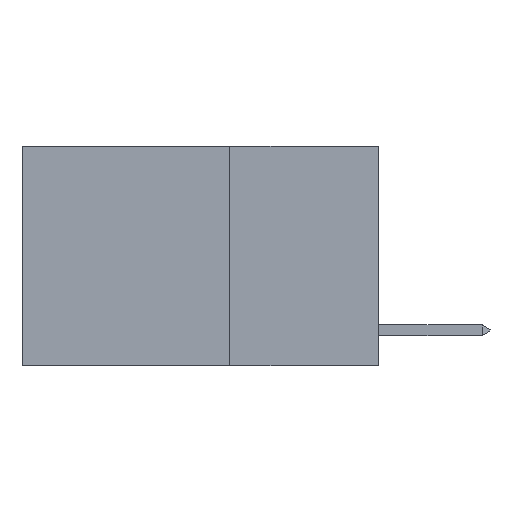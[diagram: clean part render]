
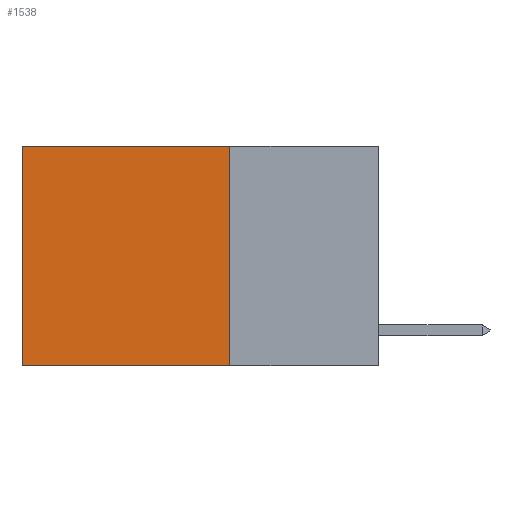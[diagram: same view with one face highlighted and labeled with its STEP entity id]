
A CAD part, left-side view. The second image highlights one B-rep face of the part: STEP entity #1538.
In plain terms, the highlighted planar face has unit normal (-1, 0, 0).
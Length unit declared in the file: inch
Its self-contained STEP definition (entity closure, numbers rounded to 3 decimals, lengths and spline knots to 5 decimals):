
#227 = CARTESIAN_POINT ( 'NONE',  ( 0.2625, 0.25, -0.37 ) ) ;
#251 = LINE ( 'NONE', #4106, #9109 ) ;
#510 = EDGE_CURVE ( 'NONE', #10621, #9238, #251, .T. ) ;
#785 = ORIENTED_EDGE ( 'NONE', *, *, #6155, .F. ) ;
#881 = DIRECTION ( 'NONE',  ( 0., 1., 0. ) ) ;
#1081 = LINE ( 'NONE', #10365, #2704 ) ;
#1084 = VERTEX_POINT ( 'NONE', #8723 ) ;
#1538 = ADVANCED_FACE ( 'NONE', ( #9565 ), #6943, .F. ) ;
#2236 = VECTOR ( 'NONE', #9667, 39.37008 ) ;
#2458 = LINE ( 'NONE', #8044, #3134 ) ;
#2628 = AXIS2_PLACEMENT_3D ( 'NONE', #7135, #2821, #6001 ) ;
#2704 = VECTOR ( 'NONE', #881, 39.37008 ) ;
#2821 = DIRECTION ( 'NONE',  ( 1., 0., 0. ) ) ;
#3134 = VECTOR ( 'NONE', #11124, 39.37008 ) ;
#3176 = EDGE_CURVE ( 'NONE', #6119, #1084, #2458, .T. ) ;
#4106 = CARTESIAN_POINT ( 'NONE',  ( 0.2625, 0.6, 0. ) ) ;
#5242 = ORIENTED_EDGE ( 'NONE', *, *, #6994, .T. ) ;
#6001 = DIRECTION ( 'NONE',  ( 0., 0., -1. ) ) ;
#6119 = VERTEX_POINT ( 'NONE', #10508 ) ;
#6155 = EDGE_CURVE ( 'NONE', #1084, #9238, #13558, .T. ) ;
#6943 = PLANE ( 'NONE',  #2628 ) ;
#6994 = EDGE_CURVE ( 'NONE', #6119, #10621, #1081, .T. ) ;
#7135 = CARTESIAN_POINT ( 'NONE',  ( 0.2625, 0.25, 0. ) ) ;
#7922 = ORIENTED_EDGE ( 'NONE', *, *, #510, .T. ) ;
#8044 = CARTESIAN_POINT ( 'NONE',  ( 0.2625, 0.25, 0. ) ) ;
#8723 = CARTESIAN_POINT ( 'NONE',  ( 0.2625, 0.25, -0.37 ) ) ;
#8806 = EDGE_LOOP ( 'NONE', ( #7922, #785, #10572, #5242 ) ) ;
#9109 = VECTOR ( 'NONE', #12484, 39.37008 ) ;
#9238 = VERTEX_POINT ( 'NONE', #9365 ) ;
#9365 = CARTESIAN_POINT ( 'NONE',  ( 0.2625, 0.6, -0.37 ) ) ;
#9565 = FACE_OUTER_BOUND ( 'NONE', #8806, .T. ) ;
#9667 = DIRECTION ( 'NONE',  ( 0., 1., 0. ) ) ;
#10365 = CARTESIAN_POINT ( 'NONE',  ( 0.2625, 0.25, 0. ) ) ;
#10508 = CARTESIAN_POINT ( 'NONE',  ( 0.2625, 0.25, 0. ) ) ;
#10572 = ORIENTED_EDGE ( 'NONE', *, *, #3176, .F. ) ;
#10621 = VERTEX_POINT ( 'NONE', #12940 ) ;
#11124 = DIRECTION ( 'NONE',  ( 0., 0., -1. ) ) ;
#12484 = DIRECTION ( 'NONE',  ( 0., 0., -1. ) ) ;
#12940 = CARTESIAN_POINT ( 'NONE',  ( 0.2625, 0.6, 0. ) ) ;
#13558 = LINE ( 'NONE', #227, #2236 ) ;
